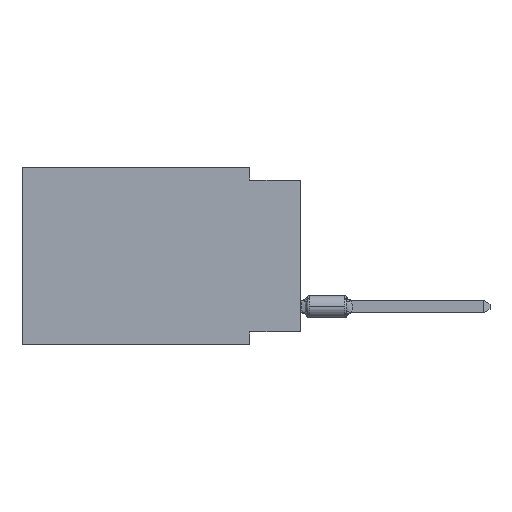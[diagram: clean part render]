
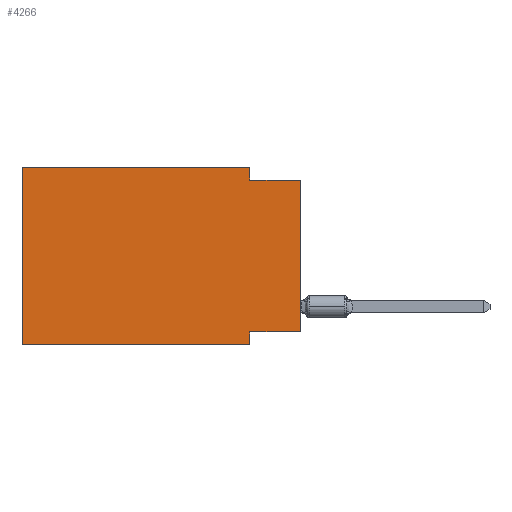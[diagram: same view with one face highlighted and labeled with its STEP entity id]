
A CAD part, left-side view. The second image highlights one B-rep face of the part: STEP entity #4266.
In plain terms, the highlighted planar face has unit normal (-1, 0, 0).
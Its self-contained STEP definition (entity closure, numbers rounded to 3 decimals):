
#280 = ORIENTED_EDGE ( 'NONE', *, *, #5061, .T. ) ;
#383 = ORIENTED_EDGE ( 'NONE', *, *, #7259, .F. ) ;
#534 = ORIENTED_EDGE ( 'NONE', *, *, #14134, .F. ) ;
#540 = VECTOR ( 'NONE', #7646, 1000. ) ;
#566 = LINE ( 'NONE', #15454, #13461 ) ;
#627 = EDGE_CURVE ( 'NONE', #10115, #4687, #4703, .T. ) ;
#641 = VECTOR ( 'NONE', #732, 1000. ) ;
#732 = DIRECTION ( 'NONE',  ( 0., -1., 0. ) ) ;
#883 = CARTESIAN_POINT ( 'NONE',  ( 0., 0., -0.635 ) ) ;
#1266 = EDGE_CURVE ( 'NONE', #14295, #3919, #1690, .T. ) ;
#1422 = VERTEX_POINT ( 'NONE', #4300 ) ;
#1690 = LINE ( 'NONE', #15971, #12186 ) ;
#1770 = ORIENTED_EDGE ( 'NONE', *, *, #5892, .F. ) ;
#1969 = ORIENTED_EDGE ( 'NONE', *, *, #10150, .T. ) ;
#2091 = CARTESIAN_POINT ( 'NONE',  ( 0., 13.97, -8.89 ) ) ;
#2486 = CARTESIAN_POINT ( 'NONE',  ( 0., 13.97, 0. ) ) ;
#2636 = LINE ( 'NONE', #14151, #540 ) ;
#3346 = ORIENTED_EDGE ( 'NONE', *, *, #10367, .F. ) ;
#3919 = VERTEX_POINT ( 'NONE', #16527 ) ;
#4266 = ADVANCED_FACE ( 'NONE', ( #10008 ), #11350, .F. ) ;
#4300 = CARTESIAN_POINT ( 'NONE',  ( 0., 0., -0.635 ) ) ;
#4479 = CARTESIAN_POINT ( 'NONE',  ( 0., 0., -8.255 ) ) ;
#4506 = AXIS2_PLACEMENT_3D ( 'NONE', #2486, #11439, #16509 ) ;
#4687 = VERTEX_POINT ( 'NONE', #9937 ) ;
#4703 = LINE ( 'NONE', #6956, #8167 ) ;
#4825 = VERTEX_POINT ( 'NONE', #13083 ) ;
#4851 = EDGE_LOOP ( 'NONE', ( #280, #3346, #16260, #534, #1770, #1969, #383, #11459 ) ) ;
#5061 = EDGE_CURVE ( 'NONE', #14295, #1422, #10601, .T. ) ;
#5721 = CARTESIAN_POINT ( 'NONE',  ( 0., 2.54, -8.89 ) ) ;
#5892 = EDGE_CURVE ( 'NONE', #6555, #4825, #2636, .T. ) ;
#5999 = CARTESIAN_POINT ( 'NONE',  ( 0., 13.97, 0. ) ) ;
#6555 = VERTEX_POINT ( 'NONE', #2091 ) ;
#6770 = CARTESIAN_POINT ( 'NONE',  ( 0., 0., 0. ) ) ;
#6956 = CARTESIAN_POINT ( 'NONE',  ( 0., 2.54, 0. ) ) ;
#6971 = DIRECTION ( 'NONE',  ( 0., 1., 0. ) ) ;
#7071 = VECTOR ( 'NONE', #13611, 1000. ) ;
#7118 = DIRECTION ( 'NONE',  ( 0., 0., -1. ) ) ;
#7259 = EDGE_CURVE ( 'NONE', #3919, #9887, #14486, .T. ) ;
#7646 = DIRECTION ( 'NONE',  ( 0., 0., 1. ) ) ;
#8167 = VECTOR ( 'NONE', #7118, 1000. ) ;
#8342 = LINE ( 'NONE', #883, #641 ) ;
#8749 = LINE ( 'NONE', #5999, #7071 ) ;
#8771 = VECTOR ( 'NONE', #11468, 1000. ) ;
#8854 = VECTOR ( 'NONE', #14569, 1000. ) ;
#9887 = VERTEX_POINT ( 'NONE', #5721 ) ;
#9937 = CARTESIAN_POINT ( 'NONE',  ( 0., 2.54, -0.635 ) ) ;
#10008 = FACE_OUTER_BOUND ( 'NONE', #4851, .T. ) ;
#10115 = VERTEX_POINT ( 'NONE', #13965 ) ;
#10150 = EDGE_CURVE ( 'NONE', #6555, #9887, #566, .T. ) ;
#10367 = EDGE_CURVE ( 'NONE', #4687, #1422, #8342, .T. ) ;
#10601 = LINE ( 'NONE', #6770, #8771 ) ;
#11350 = PLANE ( 'NONE',  #4506 ) ;
#11439 = DIRECTION ( 'NONE',  ( 1., 0., 0. ) ) ;
#11459 = ORIENTED_EDGE ( 'NONE', *, *, #1266, .F. ) ;
#11468 = DIRECTION ( 'NONE',  ( 0., 0., 1. ) ) ;
#12186 = VECTOR ( 'NONE', #6971, 1000. ) ;
#13083 = CARTESIAN_POINT ( 'NONE',  ( 0., 13.97, 0. ) ) ;
#13342 = CARTESIAN_POINT ( 'NONE',  ( 0., 2.54, -8.89 ) ) ;
#13461 = VECTOR ( 'NONE', #14046, 1000. ) ;
#13611 = DIRECTION ( 'NONE',  ( 0., -1., 0. ) ) ;
#13965 = CARTESIAN_POINT ( 'NONE',  ( 0., 2.54, 0. ) ) ;
#14046 = DIRECTION ( 'NONE',  ( 0., -1., 0. ) ) ;
#14134 = EDGE_CURVE ( 'NONE', #4825, #10115, #8749, .T. ) ;
#14151 = CARTESIAN_POINT ( 'NONE',  ( 0., 13.97, 0. ) ) ;
#14295 = VERTEX_POINT ( 'NONE', #4479 ) ;
#14486 = LINE ( 'NONE', #13342, #8854 ) ;
#14569 = DIRECTION ( 'NONE',  ( 0., 0., -1. ) ) ;
#15454 = CARTESIAN_POINT ( 'NONE',  ( 0., 13.97, -8.89 ) ) ;
#15971 = CARTESIAN_POINT ( 'NONE',  ( 0., 0., -8.255 ) ) ;
#16260 = ORIENTED_EDGE ( 'NONE', *, *, #627, .F. ) ;
#16509 = DIRECTION ( 'NONE',  ( 0., 0., -1. ) ) ;
#16527 = CARTESIAN_POINT ( 'NONE',  ( 0., 2.54, -8.255 ) ) ;
